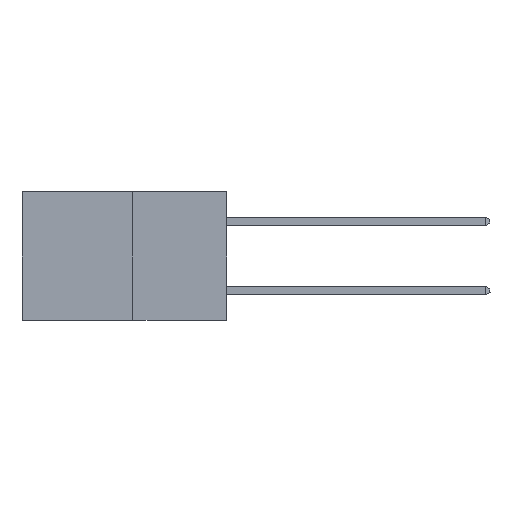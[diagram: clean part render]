
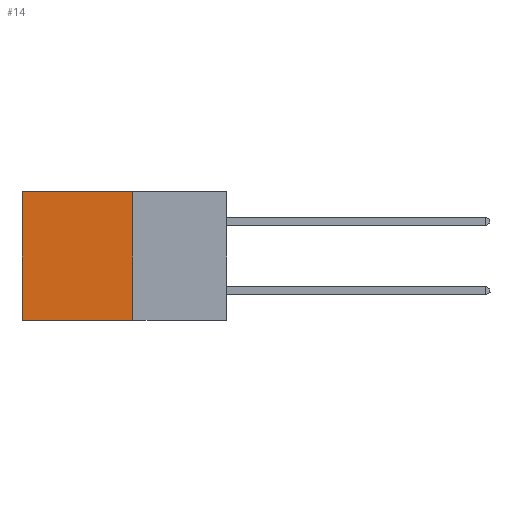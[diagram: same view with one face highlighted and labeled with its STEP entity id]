
A CAD part, left-side view. The second image highlights one B-rep face of the part: STEP entity #14.
In plain terms, the highlighted planar face has unit normal (-1, 0, 0).
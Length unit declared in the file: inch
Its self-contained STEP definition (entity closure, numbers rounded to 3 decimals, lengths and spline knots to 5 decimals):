
#14 = ADVANCED_FACE ( 'NONE', ( #13144 ), #9843, .F. ) ;
#2203 = VERTEX_POINT ( 'NONE', #18592 ) ;
#2421 = ORIENTED_EDGE ( 'NONE', *, *, #22651, .F. ) ;
#2511 = CARTESIAN_POINT ( 'NONE',  ( 0.277, 0.27, -0.37 ) ) ;
#2948 = DIRECTION ( 'NONE',  ( 0., 1., 0. ) ) ;
#3070 = ORIENTED_EDGE ( 'NONE', *, *, #30813, .F. ) ;
#4106 = CARTESIAN_POINT ( 'NONE',  ( 0.277, 0.27, -0.37 ) ) ;
#5457 = DIRECTION ( 'NONE',  ( 0., 0., -1. ) ) ;
#5750 = ORIENTED_EDGE ( 'NONE', *, *, #31188, .T. ) ;
#6351 = VECTOR ( 'NONE', #9398, 39.37008 ) ;
#7165 = LINE ( 'NONE', #4106, #6351 ) ;
#7763 = CARTESIAN_POINT ( 'NONE',  ( 0.277, 0.27, -0.37 ) ) ;
#8355 = VERTEX_POINT ( 'NONE', #21793 ) ;
#8775 = VERTEX_POINT ( 'NONE', #31870 ) ;
#9398 = DIRECTION ( 'NONE',  ( 0., 1., 0. ) ) ;
#9810 = DIRECTION ( 'NONE',  ( 1., 0., 0. ) ) ;
#9843 = PLANE ( 'NONE',  #29377 ) ;
#11355 = EDGE_LOOP ( 'NONE', ( #5750, #3070, #2421, #28321 ) ) ;
#13144 = FACE_OUTER_BOUND ( 'NONE', #11355, .T. ) ;
#15380 = CARTESIAN_POINT ( 'NONE',  ( 0.277, 0.27, 0. ) ) ;
#15993 = VECTOR ( 'NONE', #23166, 39.37008 ) ;
#16596 = VECTOR ( 'NONE', #2948, 39.37008 ) ;
#18180 = VERTEX_POINT ( 'NONE', #15380 ) ;
#18258 = EDGE_CURVE ( 'NONE', #18180, #8355, #30960, .T. ) ;
#18592 = CARTESIAN_POINT ( 'NONE',  ( 0.277, 0.27, -0.37 ) ) ;
#21028 = CARTESIAN_POINT ( 'NONE',  ( 0.277, 0.27, 0. ) ) ;
#21669 = LINE ( 'NONE', #23685, #27659 ) ;
#21793 = CARTESIAN_POINT ( 'NONE',  ( 0.277, 0.59, 0. ) ) ;
#22651 = EDGE_CURVE ( 'NONE', #18180, #2203, #22813, .T. ) ;
#22813 = LINE ( 'NONE', #2511, #15993 ) ;
#23166 = DIRECTION ( 'NONE',  ( 0., 0., -1. ) ) ;
#23685 = CARTESIAN_POINT ( 'NONE',  ( 0.277, 0.59, -0.37 ) ) ;
#26240 = DIRECTION ( 'NONE',  ( 0., 0., -1. ) ) ;
#27659 = VECTOR ( 'NONE', #26240, 39.37008 ) ;
#28321 = ORIENTED_EDGE ( 'NONE', *, *, #18258, .T. ) ;
#29377 = AXIS2_PLACEMENT_3D ( 'NONE', #7763, #9810, #5457 ) ;
#30813 = EDGE_CURVE ( 'NONE', #2203, #8775, #7165, .T. ) ;
#30960 = LINE ( 'NONE', #21028, #16596 ) ;
#31188 = EDGE_CURVE ( 'NONE', #8355, #8775, #21669, .T. ) ;
#31870 = CARTESIAN_POINT ( 'NONE',  ( 0.277, 0.59, -0.37 ) ) ;
